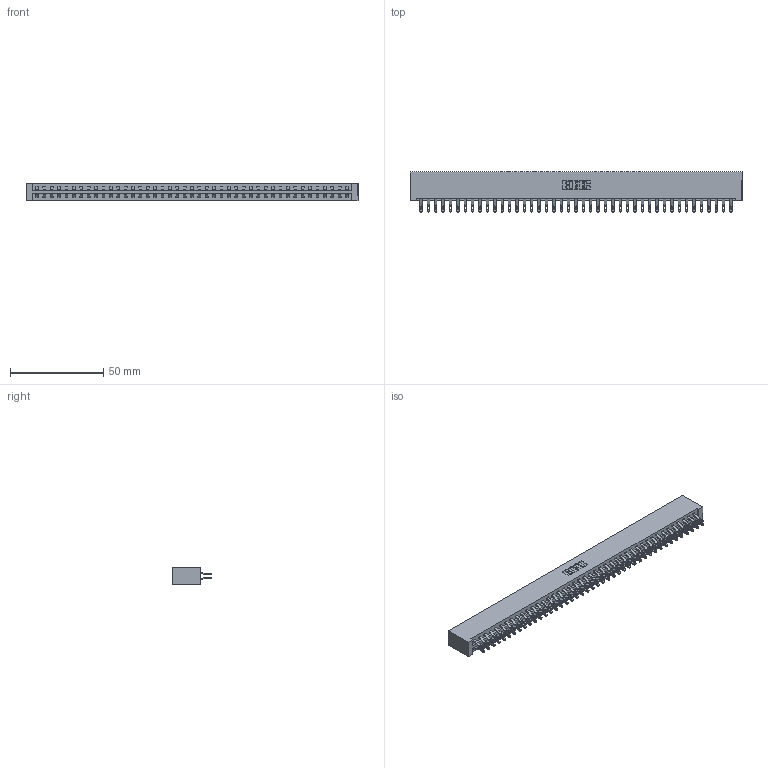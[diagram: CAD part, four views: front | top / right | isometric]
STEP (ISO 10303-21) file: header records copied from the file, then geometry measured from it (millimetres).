
FILE_DESCRIPTION (( 'STEP AP203' ), '1' );
FILE_NAME ('387-086-555-201.STEP', '2019-10-23T04:02:15', ( '' ), ( '' ), 'SwSTEP 2.0', 'SolidWorks 2016', '' );
FILE_SCHEMA (( 'CONFIG_CONTROL_DESIGN' ));
Length unit declared in the file: inch
Products named in the file (3): 337 Part_No Mounting Lugs; 387-086-555-201; 345-292-001_555 Tail
Assembly tree (87 placements, depth 2):
  387-086-555-201
    337 Part_No Mounting Lugs
    345-292-001_555 Tail  x86
Bounding box: 178.26 x 21.47 x 9.4 mm (x, y, z)
Volume: 19809.6 mm3; surface area: 23400.7 mm2
Topology: 87 solids, 87 shells, 5266 faces, 16541 edges, 11026 vertices
Faces by surface type: plane 3162, cylinder 2104
Entity records: 33259 total; most frequent: CARTESIAN_POINT 5636, ORIENTED_EDGE 5542, DIRECTION 4755, EDGE_CURVE 2771, VECTOR 2631, LINE 2631, VERTEX_POINT 1846, AXIS2_PLACEMENT_3D 1062
